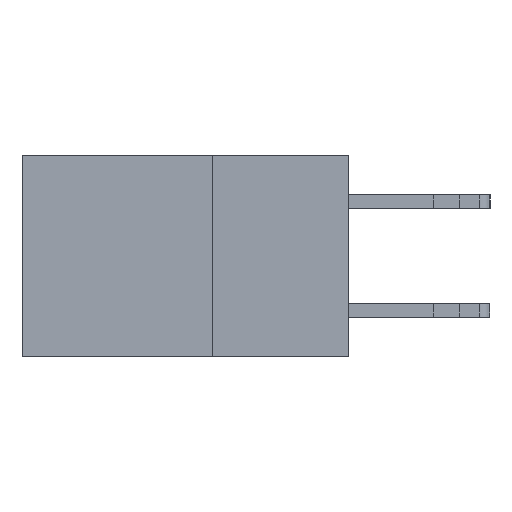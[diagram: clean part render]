
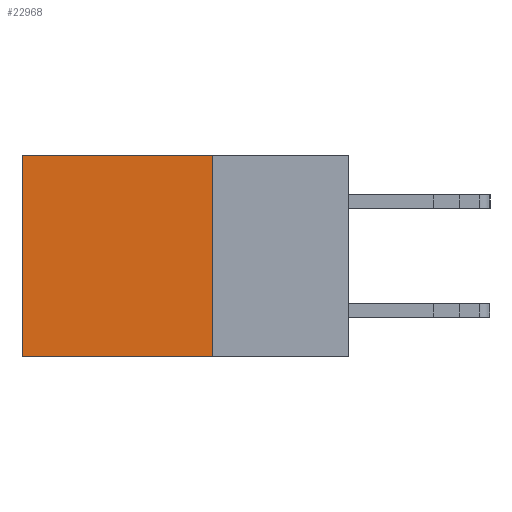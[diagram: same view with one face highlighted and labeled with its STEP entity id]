
A CAD part, left-side view. The second image highlights one B-rep face of the part: STEP entity #22968.
In plain terms, the highlighted planar face has unit normal (-1, 0, 0).
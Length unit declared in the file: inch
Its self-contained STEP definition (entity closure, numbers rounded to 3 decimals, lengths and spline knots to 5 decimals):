
#500 = VERTEX_POINT ( 'NONE', #8331 ) ;
#1470 = VECTOR ( 'NONE', #18647, 39.37008 ) ;
#1576 = VERTEX_POINT ( 'NONE', #15554 ) ;
#1897 = VECTOR ( 'NONE', #19304, 39.37008 ) ;
#1941 = EDGE_CURVE ( 'NONE', #500, #1576, #23166, .T. ) ;
#3929 = VERTEX_POINT ( 'NONE', #21394 ) ;
#5353 = AXIS2_PLACEMENT_3D ( 'NONE', #11518, #25571, #13562 ) ;
#5984 = ORIENTED_EDGE ( 'NONE', *, *, #18631, .T. ) ;
#7004 = DIRECTION ( 'NONE',  ( 0., 1., 0. ) ) ;
#7435 = VECTOR ( 'NONE', #7004, 39.37008 ) ;
#7788 = ORIENTED_EDGE ( 'NONE', *, *, #17454, .F. ) ;
#8331 = CARTESIAN_POINT ( 'NONE',  ( 0.298, 0.25, 0. ) ) ;
#8432 = DIRECTION ( 'NONE',  ( 0., 0., -1. ) ) ;
#9839 = VECTOR ( 'NONE', #8432, 39.37008 ) ;
#9941 = FACE_OUTER_BOUND ( 'NONE', #12810, .T. ) ;
#11518 = CARTESIAN_POINT ( 'NONE',  ( 0.298, 0.25, 0. ) ) ;
#11854 = CARTESIAN_POINT ( 'NONE',  ( 0.298, 0.25, 0. ) ) ;
#12174 = ORIENTED_EDGE ( 'NONE', *, *, #25151, .F. ) ;
#12810 = EDGE_LOOP ( 'NONE', ( #5984, #12174, #7788, #15845 ) ) ;
#13562 = DIRECTION ( 'NONE',  ( 0., 0., -1. ) ) ;
#14276 = VERTEX_POINT ( 'NONE', #22831 ) ;
#15182 = LINE ( 'NONE', #22423, #9839 ) ;
#15554 = CARTESIAN_POINT ( 'NONE',  ( 0.298, 0.6, 0. ) ) ;
#15845 = ORIENTED_EDGE ( 'NONE', *, *, #1941, .T. ) ;
#16665 = CARTESIAN_POINT ( 'NONE',  ( 0.298, 0.25, 0. ) ) ;
#17397 = PLANE ( 'NONE',  #5353 ) ;
#17454 = EDGE_CURVE ( 'NONE', #500, #3929, #22749, .T. ) ;
#18059 = LINE ( 'NONE', #24950, #7435 ) ;
#18631 = EDGE_CURVE ( 'NONE', #1576, #14276, #15182, .T. ) ;
#18647 = DIRECTION ( 'NONE',  ( 0., 0., -1. ) ) ;
#19304 = DIRECTION ( 'NONE',  ( 0., 1., 0. ) ) ;
#21394 = CARTESIAN_POINT ( 'NONE',  ( 0.298, 0.25, -0.37 ) ) ;
#22423 = CARTESIAN_POINT ( 'NONE',  ( 0.298, 0.6, 0. ) ) ;
#22749 = LINE ( 'NONE', #16665, #1470 ) ;
#22831 = CARTESIAN_POINT ( 'NONE',  ( 0.298, 0.6, -0.37 ) ) ;
#22968 = ADVANCED_FACE ( 'NONE', ( #9941 ), #17397, .F. ) ;
#23166 = LINE ( 'NONE', #11854, #1897 ) ;
#24950 = CARTESIAN_POINT ( 'NONE',  ( 0.298, 0.25, -0.37 ) ) ;
#25151 = EDGE_CURVE ( 'NONE', #3929, #14276, #18059, .T. ) ;
#25571 = DIRECTION ( 'NONE',  ( 1., 0., 0. ) ) ;
